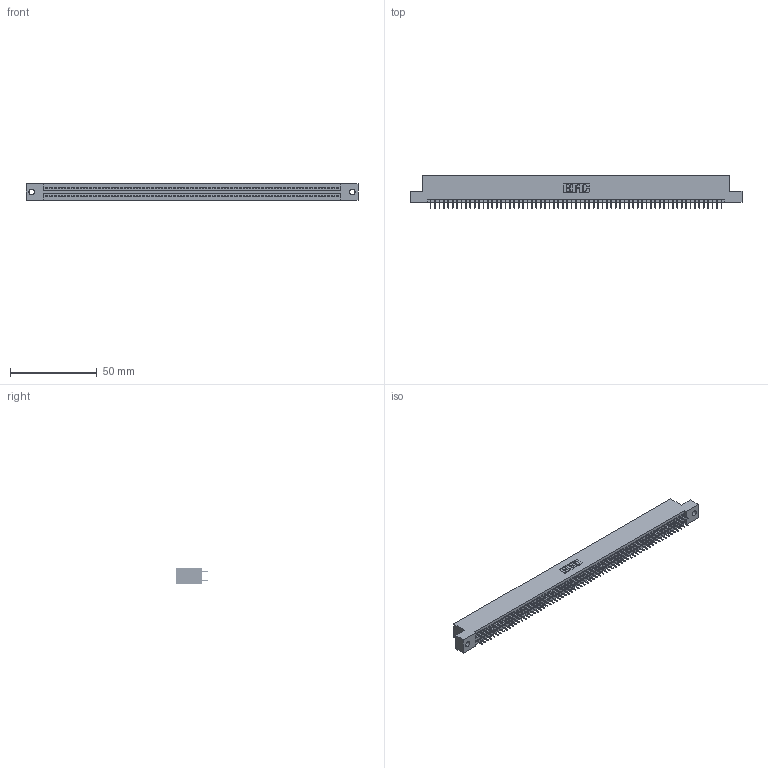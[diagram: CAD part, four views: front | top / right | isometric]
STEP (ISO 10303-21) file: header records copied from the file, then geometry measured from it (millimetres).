
FILE_DESCRIPTION (( 'STEP AP203' ), '1' );
FILE_NAME ('395-134-525-202.STEP', '2020-09-26T03:04:14', ( '' ), ( '' ), 'SwSTEP 2.0', 'SolidWorks 2020', '' );
FILE_SCHEMA (( 'CONFIG_CONTROL_DESIGN' ));
Length unit declared in the file: inch
Products named in the file (3): 345-292-001_345-293-125; 345 Part_Flush Mounting Lugs - 0.128 Dia; 395-134-525-202
Assembly tree (135 placements, depth 2):
  395-134-525-202
    345 Part_Flush Mounting Lugs - 0.128 Dia
    345-292-001_345-293-125  x134
Bounding box: 191.39 x 18.72 x 9.4 mm (x, y, z)
Volume: 18566.5 mm3; surface area: 26991.3 mm2
Topology: 135 solids, 135 shells, 7362 faces, 20843 edges, 13358 vertices
Faces by surface type: plane 5306, cylinder 2056
Entity records: 49281 total; most frequent: CARTESIAN_POINT 8236, ORIENTED_EDGE 8170, DIRECTION 7233, EDGE_CURVE 4085, LINE 3689, VECTOR 3689, VERTEX_POINT 2718, AXIS2_PLACEMENT_3D 1772
